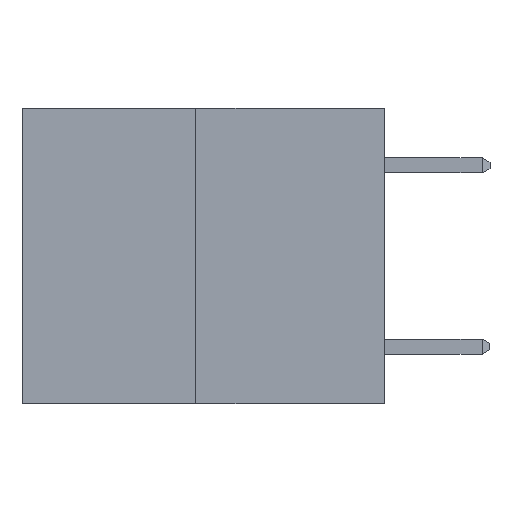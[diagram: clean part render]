
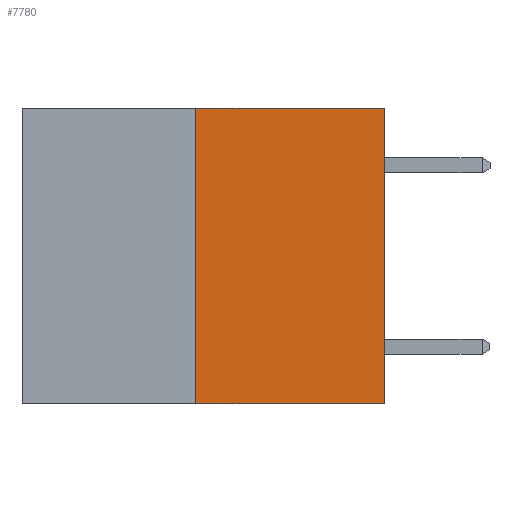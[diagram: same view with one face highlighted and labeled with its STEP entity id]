
A CAD part, left-side view. The second image highlights one B-rep face of the part: STEP entity #7780.
In plain terms, the highlighted planar face has unit normal (-1, 0, 0).
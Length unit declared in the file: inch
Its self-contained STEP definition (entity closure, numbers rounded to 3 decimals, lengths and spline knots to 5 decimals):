
#721 = VECTOR ( 'NONE', #2856, 39.37008 ) ;
#887 = EDGE_CURVE ( 'NONE', #4617, #12603, #5741, .T. ) ;
#1372 = VECTOR ( 'NONE', #6569, 39.37008 ) ;
#1565 = EDGE_CURVE ( 'NONE', #13648, #12603, #7718, .T. ) ;
#1626 = ORIENTED_EDGE ( 'NONE', *, *, #3301, .F. ) ;
#1877 = ORIENTED_EDGE ( 'NONE', *, *, #887, .F. ) ;
#1946 = VERTEX_POINT ( 'NONE', #10045 ) ;
#2856 = DIRECTION ( 'NONE',  ( 0., 0., 1. ) ) ;
#3073 = PLANE ( 'NONE',  #6045 ) ;
#3301 = EDGE_CURVE ( 'NONE', #1946, #4617, #9084, .T. ) ;
#4408 = EDGE_CURVE ( 'NONE', #1946, #13648, #4618, .T. ) ;
#4617 = VERTEX_POINT ( 'NONE', #10727 ) ;
#4618 = LINE ( 'NONE', #6016, #7517 ) ;
#4863 = DIRECTION ( 'NONE',  ( 0., -1., 0. ) ) ;
#5230 = CARTESIAN_POINT ( 'NONE',  ( 0., 0.6, 0. ) ) ;
#5741 = LINE ( 'NONE', #5230, #9524 ) ;
#6016 = CARTESIAN_POINT ( 'NONE',  ( 0., 0.6, -0.49 ) ) ;
#6045 = AXIS2_PLACEMENT_3D ( 'NONE', #10090, #10133, #11091 ) ;
#6569 = DIRECTION ( 'NONE',  ( 0., 0., 1. ) ) ;
#7192 = EDGE_LOOP ( 'NONE', ( #1626, #13806, #11976, #1877 ) ) ;
#7517 = VECTOR ( 'NONE', #4863, 39.37008 ) ;
#7615 = FACE_OUTER_BOUND ( 'NONE', #7192, .T. ) ;
#7718 = LINE ( 'NONE', #9989, #1372 ) ;
#7780 = ADVANCED_FACE ( 'NONE', ( #7615 ), #3073, .F. ) ;
#9084 = LINE ( 'NONE', #14376, #721 ) ;
#9524 = VECTOR ( 'NONE', #13390, 39.37008 ) ;
#9989 = CARTESIAN_POINT ( 'NONE',  ( 0., 0., 0. ) ) ;
#10045 = CARTESIAN_POINT ( 'NONE',  ( 0., 0.312, -0.49 ) ) ;
#10090 = CARTESIAN_POINT ( 'NONE',  ( 0., 0.6, 0. ) ) ;
#10133 = DIRECTION ( 'NONE',  ( 1., 0., 0. ) ) ;
#10727 = CARTESIAN_POINT ( 'NONE',  ( 0., 0.312, 0. ) ) ;
#11091 = DIRECTION ( 'NONE',  ( 0., 0., -1. ) ) ;
#11976 = ORIENTED_EDGE ( 'NONE', *, *, #1565, .T. ) ;
#12603 = VERTEX_POINT ( 'NONE', #13332 ) ;
#13332 = CARTESIAN_POINT ( 'NONE',  ( 0., 0., 0. ) ) ;
#13390 = DIRECTION ( 'NONE',  ( 0., -1., 0. ) ) ;
#13648 = VERTEX_POINT ( 'NONE', #13750 ) ;
#13750 = CARTESIAN_POINT ( 'NONE',  ( 0., 0., -0.49 ) ) ;
#13806 = ORIENTED_EDGE ( 'NONE', *, *, #4408, .T. ) ;
#14376 = CARTESIAN_POINT ( 'NONE',  ( 0., 0.312, -0.49 ) ) ;
